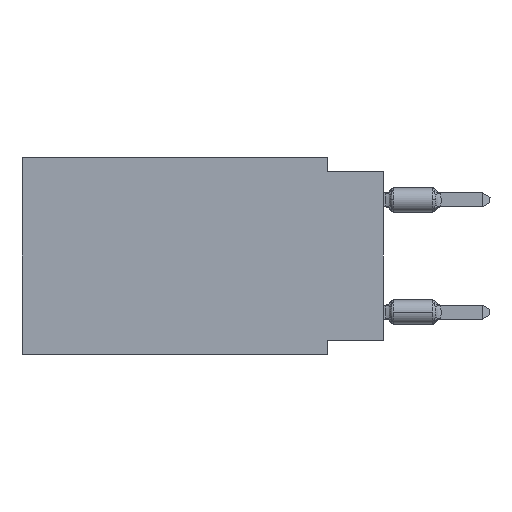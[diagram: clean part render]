
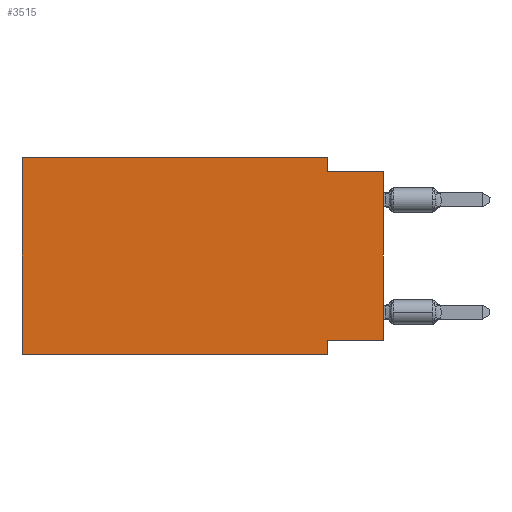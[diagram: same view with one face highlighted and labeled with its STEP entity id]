
A CAD part, left-side view. The second image highlights one B-rep face of the part: STEP entity #3515.
In plain terms, the highlighted planar face has unit normal (-1, 0, 0).
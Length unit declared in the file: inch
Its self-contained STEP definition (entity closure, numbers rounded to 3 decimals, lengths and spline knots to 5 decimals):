
#105 = EDGE_CURVE ( 'NONE', #2357, #14540, #8261, .T. ) ;
#123 = ORIENTED_EDGE ( 'NONE', *, *, #105, .F. ) ;
#318 = LINE ( 'NONE', #14444, #15032 ) ;
#377 = LINE ( 'NONE', #13294, #8769 ) ;
#2124 = LINE ( 'NONE', #7782, #13829 ) ;
#2357 = VERTEX_POINT ( 'NONE', #14429 ) ;
#2667 = CARTESIAN_POINT ( 'NONE',  ( 0., 0.645, -0.35 ) ) ;
#3109 = CARTESIAN_POINT ( 'NONE',  ( 0., 0.1, -0.35 ) ) ;
#3202 = CARTESIAN_POINT ( 'NONE',  ( 0., 0.645, 0. ) ) ;
#3239 = DIRECTION ( 'NONE',  ( 0., 0., 1. ) ) ;
#3459 = LINE ( 'NONE', #3202, #6693 ) ;
#3515 = ADVANCED_FACE ( 'NONE', ( #13360 ), #17714, .F. ) ;
#3544 = CARTESIAN_POINT ( 'NONE',  ( 0., 0., -0.025 ) ) ;
#3943 = CARTESIAN_POINT ( 'NONE',  ( 0., 0.1, -0.025 ) ) ;
#4646 = DIRECTION ( 'NONE',  ( 0., -1., 0. ) ) ;
#4798 = ORIENTED_EDGE ( 'NONE', *, *, #9245, .F. ) ;
#5160 = EDGE_CURVE ( 'NONE', #11303, #6199, #7656, .T. ) ;
#5579 = CARTESIAN_POINT ( 'NONE',  ( 0., 0., -0.325 ) ) ;
#5606 = DIRECTION ( 'NONE',  ( 0., 0., 1. ) ) ;
#6009 = CARTESIAN_POINT ( 'NONE',  ( 0., 0.645, -0.35 ) ) ;
#6199 = VERTEX_POINT ( 'NONE', #3943 ) ;
#6202 = CARTESIAN_POINT ( 'NONE',  ( 0., 0.645, 0. ) ) ;
#6391 = DIRECTION ( 'NONE',  ( 0., 0., -1. ) ) ;
#6693 = VECTOR ( 'NONE', #17501, 39.37008 ) ;
#6842 = EDGE_CURVE ( 'NONE', #14540, #8760, #2124, .T. ) ;
#7656 = LINE ( 'NONE', #14640, #12718 ) ;
#7712 = ORIENTED_EDGE ( 'NONE', *, *, #7734, .F. ) ;
#7734 = EDGE_CURVE ( 'NONE', #15628, #11303, #3459, .T. ) ;
#7782 = CARTESIAN_POINT ( 'NONE',  ( 0., 0.1, -0.35 ) ) ;
#7981 = AXIS2_PLACEMENT_3D ( 'NONE', #6202, #16149, #16062 ) ;
#8261 = LINE ( 'NONE', #5579, #16038 ) ;
#8760 = VERTEX_POINT ( 'NONE', #3109 ) ;
#8769 = VECTOR ( 'NONE', #4646, 39.37008 ) ;
#9144 = ORIENTED_EDGE ( 'NONE', *, *, #5160, .F. ) ;
#9245 = EDGE_CURVE ( 'NONE', #6199, #9774, #377, .T. ) ;
#9443 = CARTESIAN_POINT ( 'NONE',  ( 0., 0.1, -0.325 ) ) ;
#9582 = ORIENTED_EDGE ( 'NONE', *, *, #11392, .T. ) ;
#9599 = CARTESIAN_POINT ( 'NONE',  ( 0., 0.645, 0. ) ) ;
#9774 = VERTEX_POINT ( 'NONE', #3544 ) ;
#9813 = LINE ( 'NONE', #2667, #18322 ) ;
#10425 = EDGE_CURVE ( 'NONE', #13600, #15628, #318, .T. ) ;
#10581 = ORIENTED_EDGE ( 'NONE', *, *, #11292, .T. ) ;
#11019 = DIRECTION ( 'NONE',  ( 0., -1., 0. ) ) ;
#11292 = EDGE_CURVE ( 'NONE', #13600, #8760, #9813, .T. ) ;
#11303 = VERTEX_POINT ( 'NONE', #12423 ) ;
#11392 = EDGE_CURVE ( 'NONE', #2357, #9774, #15693, .T. ) ;
#11682 = ORIENTED_EDGE ( 'NONE', *, *, #10425, .F. ) ;
#12423 = CARTESIAN_POINT ( 'NONE',  ( 0., 0.1, 0. ) ) ;
#12718 = VECTOR ( 'NONE', #13234, 39.37008 ) ;
#13234 = DIRECTION ( 'NONE',  ( 0., 0., -1. ) ) ;
#13294 = CARTESIAN_POINT ( 'NONE',  ( 0., 0., -0.025 ) ) ;
#13360 = FACE_OUTER_BOUND ( 'NONE', #16508, .T. ) ;
#13600 = VERTEX_POINT ( 'NONE', #6009 ) ;
#13829 = VECTOR ( 'NONE', #6391, 39.37008 ) ;
#14429 = CARTESIAN_POINT ( 'NONE',  ( 0., 0., -0.325 ) ) ;
#14444 = CARTESIAN_POINT ( 'NONE',  ( 0., 0.645, 0. ) ) ;
#14540 = VERTEX_POINT ( 'NONE', #9443 ) ;
#14640 = CARTESIAN_POINT ( 'NONE',  ( 0., 0.1, 0. ) ) ;
#15032 = VECTOR ( 'NONE', #5606, 39.37008 ) ;
#15447 = DIRECTION ( 'NONE',  ( 0., 1., 0. ) ) ;
#15628 = VERTEX_POINT ( 'NONE', #9599 ) ;
#15693 = LINE ( 'NONE', #17166, #15970 ) ;
#15947 = ORIENTED_EDGE ( 'NONE', *, *, #6842, .F. ) ;
#15970 = VECTOR ( 'NONE', #3239, 39.37008 ) ;
#16038 = VECTOR ( 'NONE', #15447, 39.37008 ) ;
#16062 = DIRECTION ( 'NONE',  ( 0., 0., -1. ) ) ;
#16149 = DIRECTION ( 'NONE',  ( 1., 0., 0. ) ) ;
#16508 = EDGE_LOOP ( 'NONE', ( #9582, #4798, #9144, #7712, #11682, #10581, #15947, #123 ) ) ;
#17166 = CARTESIAN_POINT ( 'NONE',  ( 0., 0., 0. ) ) ;
#17501 = DIRECTION ( 'NONE',  ( 0., -1., 0. ) ) ;
#17714 = PLANE ( 'NONE',  #7981 ) ;
#18322 = VECTOR ( 'NONE', #11019, 39.37008 ) ;
